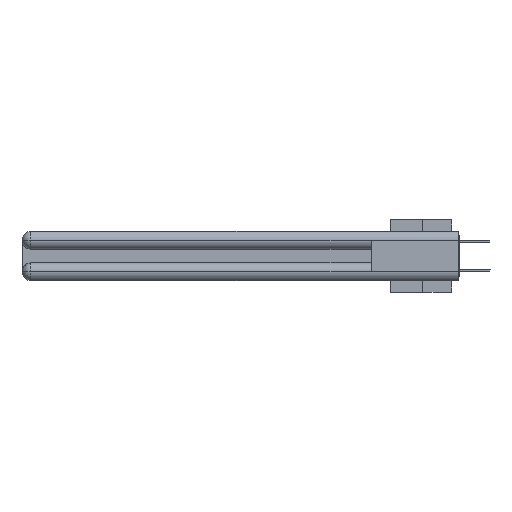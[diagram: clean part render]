
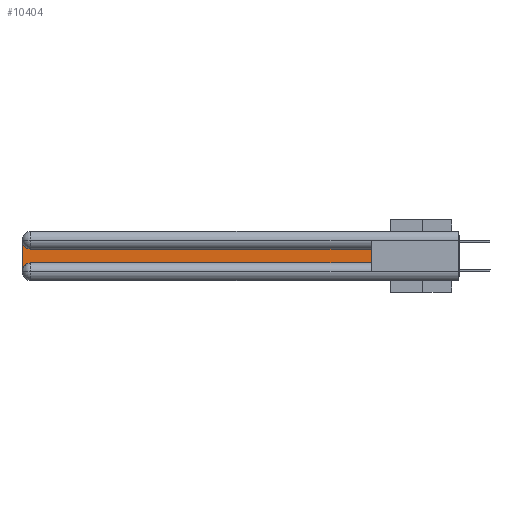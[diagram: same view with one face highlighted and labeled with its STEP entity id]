
A CAD part, left-side view. The second image highlights one B-rep face of the part: STEP entity #10404.
In plain terms, the highlighted planar face has unit normal (-1, 0, 0).
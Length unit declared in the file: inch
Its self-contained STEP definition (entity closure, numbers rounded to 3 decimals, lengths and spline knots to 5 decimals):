
#273 = EDGE_CURVE ( 'NONE', #19837, #16844, #13712, .T. ) ;
#326 = VERTEX_POINT ( 'NONE', #9916 ) ;
#733 = DIRECTION ( 'NONE',  ( 0., -1., 0. ) ) ;
#1019 = CARTESIAN_POINT ( 'NONE',  ( 0.075, 2.94, -0.1225 ) ) ;
#1260 = DIRECTION ( 'NONE',  ( 0., 0., -1. ) ) ;
#1772 = ORIENTED_EDGE ( 'NONE', *, *, #20602, .T. ) ;
#2505 = ORIENTED_EDGE ( 'NONE', *, *, #15555, .T. ) ;
#3318 = CIRCLE ( 'NONE', #8288, 0.06 ) ;
#3323 = LINE ( 'NONE', #22575, #8493 ) ;
#3876 = ORIENTED_EDGE ( 'NONE', *, *, #273, .T. ) ;
#4447 = CARTESIAN_POINT ( 'NONE',  ( 0.075, 0.6, -0.1225 ) ) ;
#4543 = CARTESIAN_POINT ( 'NONE',  ( 0.075, 3., -0.0625 ) ) ;
#4655 = DIRECTION ( 'NONE',  ( 1., 0., 0. ) ) ;
#4832 = DIRECTION ( 'NONE',  ( 0., 0., -1. ) ) ;
#6857 = ORIENTED_EDGE ( 'NONE', *, *, #24237, .T. ) ;
#6987 = VECTOR ( 'NONE', #733, 39.37008 ) ;
#7744 = CARTESIAN_POINT ( 'NONE',  ( 0.075, 0.6, -0.2175 ) ) ;
#8288 = AXIS2_PLACEMENT_3D ( 'NONE', #9058, #23327, #4832 ) ;
#8493 = VECTOR ( 'NONE', #1260, 39.37008 ) ;
#9058 = CARTESIAN_POINT ( 'NONE',  ( 0.075, 2.94, -0.2775 ) ) ;
#9331 = DIRECTION ( 'NONE',  ( 0., 0., -1. ) ) ;
#9916 = CARTESIAN_POINT ( 'NONE',  ( 0.075, 0.6, -0.2175 ) ) ;
#10062 = VERTEX_POINT ( 'NONE', #10717 ) ;
#10216 = LINE ( 'NONE', #7744, #6987 ) ;
#10351 = EDGE_CURVE ( 'NONE', #10062, #326, #10216, .T. ) ;
#10404 = ADVANCED_FACE ( 'NONE', ( #12871 ), #16906, .F. ) ;
#10717 = CARTESIAN_POINT ( 'NONE',  ( 0.075, 2.94, -0.2175 ) ) ;
#12295 = CIRCLE ( 'NONE', #20236, 0.06 ) ;
#12871 = FACE_OUTER_BOUND ( 'NONE', #28535, .T. ) ;
#13712 = LINE ( 'NONE', #27880, #24049 ) ;
#13768 = VERTEX_POINT ( 'NONE', #4543 ) ;
#15555 = EDGE_CURVE ( 'NONE', #16844, #13768, #12295, .T. ) ;
#15875 = AXIS2_PLACEMENT_3D ( 'NONE', #24695, #26874, #26556 ) ;
#16326 = EDGE_CURVE ( 'NONE', #326, #19837, #21955, .T. ) ;
#16844 = VERTEX_POINT ( 'NONE', #1019 ) ;
#16906 = PLANE ( 'NONE',  #15875 ) ;
#17136 = CARTESIAN_POINT ( 'NONE',  ( 0.075, 0.6, -0.2175 ) ) ;
#17255 = ORIENTED_EDGE ( 'NONE', *, *, #10351, .T. ) ;
#19837 = VERTEX_POINT ( 'NONE', #4447 ) ;
#19931 = DIRECTION ( 'NONE',  ( 0., 0., 1. ) ) ;
#20236 = AXIS2_PLACEMENT_3D ( 'NONE', #30643, #4655, #9331 ) ;
#20602 = EDGE_CURVE ( 'NONE', #13768, #21639, #3323, .T. ) ;
#21639 = VERTEX_POINT ( 'NONE', #30774 ) ;
#21955 = LINE ( 'NONE', #17136, #29228 ) ;
#22575 = CARTESIAN_POINT ( 'NONE',  ( 0.075, 3., -0.2175 ) ) ;
#23327 = DIRECTION ( 'NONE',  ( 1., 0., 0. ) ) ;
#23632 = ORIENTED_EDGE ( 'NONE', *, *, #16326, .T. ) ;
#24049 = VECTOR ( 'NONE', #30218, 39.37008 ) ;
#24237 = EDGE_CURVE ( 'NONE', #21639, #10062, #3318, .T. ) ;
#24695 = CARTESIAN_POINT ( 'NONE',  ( 0.075, 3., -0.1225 ) ) ;
#26556 = DIRECTION ( 'NONE',  ( 0., 0., -1. ) ) ;
#26874 = DIRECTION ( 'NONE',  ( 1., 0., 0. ) ) ;
#27880 = CARTESIAN_POINT ( 'NONE',  ( 0.075, 0.6, -0.1225 ) ) ;
#28535 = EDGE_LOOP ( 'NONE', ( #3876, #2505, #1772, #6857, #17255, #23632 ) ) ;
#29228 = VECTOR ( 'NONE', #19931, 39.37008 ) ;
#30218 = DIRECTION ( 'NONE',  ( 0., 1., 0. ) ) ;
#30643 = CARTESIAN_POINT ( 'NONE',  ( 0.075, 2.94, -0.0625 ) ) ;
#30774 = CARTESIAN_POINT ( 'NONE',  ( 0.075, 3., -0.2775 ) ) ;
